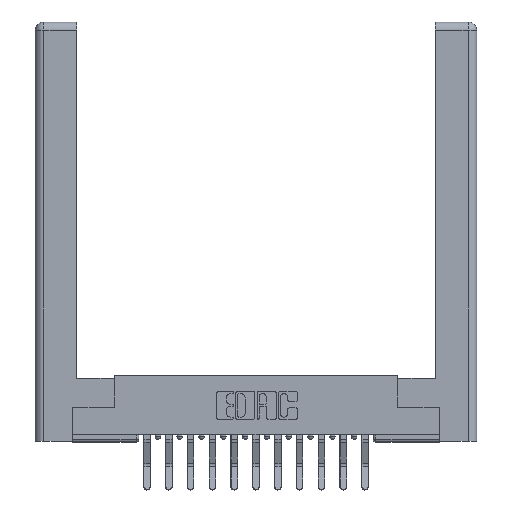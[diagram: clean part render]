
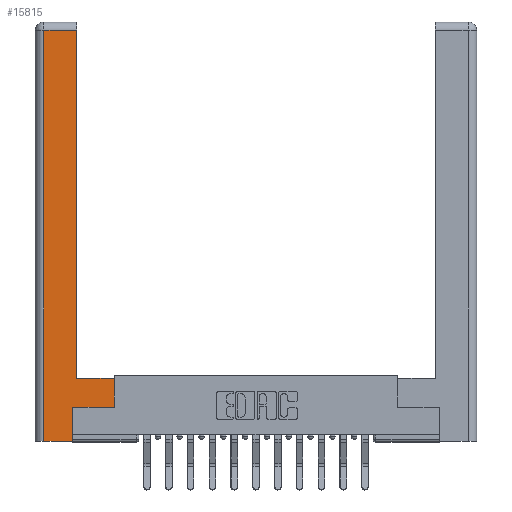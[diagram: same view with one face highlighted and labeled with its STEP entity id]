
A CAD part, top view. The second image highlights one B-rep face of the part: STEP entity #15815.
In plain terms, the highlighted planar face has unit normal (0, 0, 1).
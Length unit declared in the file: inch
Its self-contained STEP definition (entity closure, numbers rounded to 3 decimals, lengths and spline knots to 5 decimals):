
#115 = EDGE_CURVE ( 'NONE', #3886, #6123, #294, .T. ) ;
#294 = LINE ( 'NONE', #15183, #1344 ) ;
#1337 = LINE ( 'NONE', #6294, #12967 ) ;
#1344 = VECTOR ( 'NONE', #11710, 39.37008 ) ;
#1391 = EDGE_CURVE ( 'NONE', #9869, #9314, #16304, .T. ) ;
#1599 = EDGE_CURVE ( 'NONE', #11778, #9869, #9303, .T. ) ;
#1631 = EDGE_CURVE ( 'NONE', #6123, #11778, #3479, .T. ) ;
#1645 = DIRECTION ( 'NONE',  ( -1., 0., 0. ) ) ;
#1882 = ORIENTED_EDGE ( 'NONE', *, *, #5228, .T. ) ;
#2332 = EDGE_CURVE ( 'NONE', #10545, #3886, #15811, .T. ) ;
#2853 = VECTOR ( 'NONE', #12148, 39.37008 ) ;
#3410 = CARTESIAN_POINT ( 'NONE',  ( 0.265, 0.245, 0. ) ) ;
#3479 = LINE ( 'NONE', #3559, #13160 ) ;
#3559 = CARTESIAN_POINT ( 'NONE',  ( 0.265, 0., 0. ) ) ;
#3886 = VERTEX_POINT ( 'NONE', #13123 ) ;
#3978 = ORIENTED_EDGE ( 'NONE', *, *, #1631, .T. ) ;
#4112 = DIRECTION ( 'NONE',  ( -1., 0., 0. ) ) ;
#4271 = CARTESIAN_POINT ( 'NONE',  ( 0.295, 0.45, 0. ) ) ;
#4275 = ORIENTED_EDGE ( 'NONE', *, *, #10310, .T. ) ;
#4279 = CARTESIAN_POINT ( 'NONE',  ( 0.0615, 2.94, 0. ) ) ;
#4711 = LINE ( 'NONE', #9534, #7220 ) ;
#4801 = DIRECTION ( 'NONE',  ( 0., 1., 0. ) ) ;
#5084 = ORIENTED_EDGE ( 'NONE', *, *, #16001, .T. ) ;
#5228 = EDGE_CURVE ( 'NONE', #9314, #9615, #1337, .T. ) ;
#5236 = CARTESIAN_POINT ( 'NONE',  ( 0.565, 0.245, 0. ) ) ;
#6123 = VERTEX_POINT ( 'NONE', #13959 ) ;
#6294 = CARTESIAN_POINT ( 'NONE',  ( 0.565, 0.45, 0. ) ) ;
#6598 = DIRECTION ( 'NONE',  ( 0., 0., -1. ) ) ;
#7066 = ORIENTED_EDGE ( 'NONE', *, *, #1391, .T. ) ;
#7220 = VECTOR ( 'NONE', #14745, 39.37008 ) ;
#7893 = CARTESIAN_POINT ( 'NONE',  ( 0.565, 0.45, 0. ) ) ;
#8015 = CARTESIAN_POINT ( 'NONE',  ( 0.295, 2.94, 0. ) ) ;
#8178 = CARTESIAN_POINT ( 'NONE',  ( 0.565, 0.245, 0. ) ) ;
#8488 = LINE ( 'NONE', #14871, #2853 ) ;
#8621 = DIRECTION ( 'NONE',  ( 1., 0., 0. ) ) ;
#8918 = EDGE_LOOP ( 'NONE', ( #5084, #15887, #11152, #3978, #12818, #7066, #1882, #4275 ) ) ;
#9144 = DIRECTION ( 'NONE',  ( 1., 0., 0. ) ) ;
#9179 = PLANE ( 'NONE',  #11322 ) ;
#9222 = VECTOR ( 'NONE', #1645, 39.37008 ) ;
#9303 = LINE ( 'NONE', #14347, #10770 ) ;
#9314 = VERTEX_POINT ( 'NONE', #8178 ) ;
#9534 = CARTESIAN_POINT ( 'NONE',  ( 0.295, 0.45, 0. ) ) ;
#9615 = VERTEX_POINT ( 'NONE', #7893 ) ;
#9869 = VERTEX_POINT ( 'NONE', #3410 ) ;
#10310 = EDGE_CURVE ( 'NONE', #9615, #12408, #4711, .T. ) ;
#10545 = VERTEX_POINT ( 'NONE', #8015 ) ;
#10770 = VECTOR ( 'NONE', #4801, 39.37008 ) ;
#11152 = ORIENTED_EDGE ( 'NONE', *, *, #115, .T. ) ;
#11322 = AXIS2_PLACEMENT_3D ( 'NONE', #11747, #6598, #4112 ) ;
#11710 = DIRECTION ( 'NONE',  ( 0., -1., 0. ) ) ;
#11747 = CARTESIAN_POINT ( 'NONE',  ( 0., 0., 0. ) ) ;
#11778 = VERTEX_POINT ( 'NONE', #15158 ) ;
#12148 = DIRECTION ( 'NONE',  ( 0., 1., 0. ) ) ;
#12408 = VERTEX_POINT ( 'NONE', #4271 ) ;
#12818 = ORIENTED_EDGE ( 'NONE', *, *, #1599, .T. ) ;
#12967 = VECTOR ( 'NONE', #15154, 39.37008 ) ;
#13123 = CARTESIAN_POINT ( 'NONE',  ( 0.0615, 2.94, 0. ) ) ;
#13160 = VECTOR ( 'NONE', #8621, 39.37008 ) ;
#13959 = CARTESIAN_POINT ( 'NONE',  ( 0.0615, 0., 0. ) ) ;
#14347 = CARTESIAN_POINT ( 'NONE',  ( 0.265, 0.245, 0. ) ) ;
#14464 = FACE_OUTER_BOUND ( 'NONE', #8918, .T. ) ;
#14745 = DIRECTION ( 'NONE',  ( -1., 0., 0. ) ) ;
#14871 = CARTESIAN_POINT ( 'NONE',  ( 0.295, 3., 0. ) ) ;
#15154 = DIRECTION ( 'NONE',  ( 0., 1., 0. ) ) ;
#15158 = CARTESIAN_POINT ( 'NONE',  ( 0.265, 0., 0. ) ) ;
#15183 = CARTESIAN_POINT ( 'NONE',  ( 0.0615, 0., 0. ) ) ;
#15522 = VECTOR ( 'NONE', #9144, 39.37008 ) ;
#15811 = LINE ( 'NONE', #4279, #9222 ) ;
#15815 = ADVANCED_FACE ( 'NONE', ( #14464 ), #9179, .F. ) ;
#15887 = ORIENTED_EDGE ( 'NONE', *, *, #2332, .T. ) ;
#16001 = EDGE_CURVE ( 'NONE', #12408, #10545, #8488, .T. ) ;
#16304 = LINE ( 'NONE', #5236, #15522 ) ;
